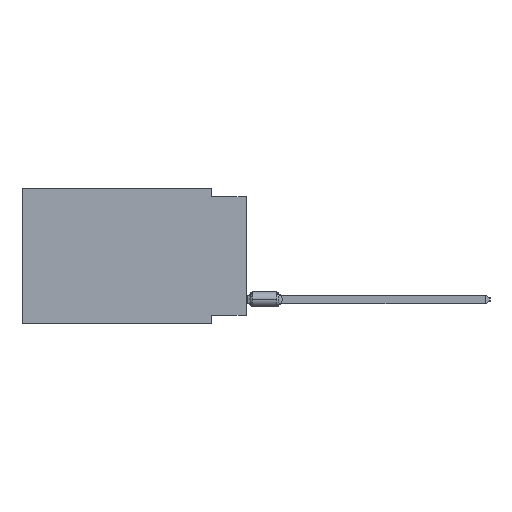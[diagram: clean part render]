
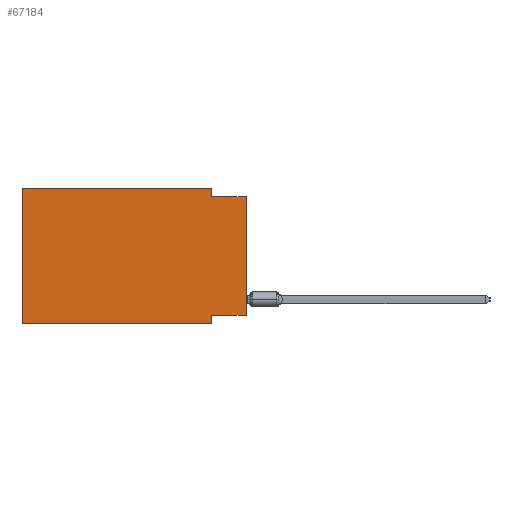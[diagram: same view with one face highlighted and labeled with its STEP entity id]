
A CAD part, left-side view. The second image highlights one B-rep face of the part: STEP entity #67184.
In plain terms, the highlighted planar face has unit normal (-1, 0, 0).
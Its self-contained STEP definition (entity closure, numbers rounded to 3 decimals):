
#1024 = VECTOR ( 'NONE', #66564, 1000. ) ;
#1289 = DIRECTION ( 'NONE',  ( 0., -1., 0. ) ) ;
#3906 = DIRECTION ( 'NONE',  ( 0., 0., -1. ) ) ;
#6473 = DIRECTION ( 'NONE',  ( 0., 0., -1. ) ) ;
#7576 = EDGE_CURVE ( 'NONE', #57149, #52475, #36486, .T. ) ;
#8618 = VECTOR ( 'NONE', #1289, 1000. ) ;
#9998 = CARTESIAN_POINT ( 'NONE',  ( 0., 2.54, -0.635 ) ) ;
#11711 = CARTESIAN_POINT ( 'NONE',  ( 0., 16.383, -9.906 ) ) ;
#12296 = CARTESIAN_POINT ( 'NONE',  ( 0., 16.383, 0. ) ) ;
#13538 = ORIENTED_EDGE ( 'NONE', *, *, #22464, .F. ) ;
#13661 = EDGE_CURVE ( 'NONE', #57149, #59132, #72105, .T. ) ;
#13826 = CARTESIAN_POINT ( 'NONE',  ( 0., 16.383, 0. ) ) ;
#14662 = VERTEX_POINT ( 'NONE', #57443 ) ;
#14938 = VERTEX_POINT ( 'NONE', #66990 ) ;
#15764 = ORIENTED_EDGE ( 'NONE', *, *, #70277, .F. ) ;
#16614 = FACE_OUTER_BOUND ( 'NONE', #52953, .T. ) ;
#16751 = ORIENTED_EDGE ( 'NONE', *, *, #29716, .T. ) ;
#17190 = CARTESIAN_POINT ( 'NONE',  ( 0., 2.54, 0. ) ) ;
#17324 = ORIENTED_EDGE ( 'NONE', *, *, #13661, .T. ) ;
#18807 = PLANE ( 'NONE',  #44376 ) ;
#18891 = EDGE_CURVE ( 'NONE', #14938, #67922, #30468, .T. ) ;
#19079 = ORIENTED_EDGE ( 'NONE', *, *, #30322, .F. ) ;
#22464 = EDGE_CURVE ( 'NONE', #52475, #14662, #55256, .T. ) ;
#22614 = CARTESIAN_POINT ( 'NONE',  ( 0., 2.54, 0. ) ) ;
#24105 = LINE ( 'NONE', #12296, #42124 ) ;
#24469 = DIRECTION ( 'NONE',  ( 0., 0., 1. ) ) ;
#26025 = VERTEX_POINT ( 'NONE', #11711 ) ;
#27175 = CARTESIAN_POINT ( 'NONE',  ( 0., 2.54, -9.906 ) ) ;
#29716 = EDGE_CURVE ( 'NONE', #26025, #14662, #68708, .T. ) ;
#30322 = EDGE_CURVE ( 'NONE', #26025, #14938, #24105, .T. ) ;
#30468 = LINE ( 'NONE', #13826, #8618 ) ;
#33229 = VECTOR ( 'NONE', #58282, 1000. ) ;
#34009 = DIRECTION ( 'NONE',  ( 0., -1., 0. ) ) ;
#34364 = CARTESIAN_POINT ( 'NONE',  ( 0., 16.383, -9.906 ) ) ;
#35000 = VECTOR ( 'NONE', #34009, 1000. ) ;
#35291 = LINE ( 'NONE', #17190, #66000 ) ;
#35441 = CARTESIAN_POINT ( 'NONE',  ( 0., 16.383, 0. ) ) ;
#35893 = VECTOR ( 'NONE', #3906, 1000. ) ;
#36170 = ORIENTED_EDGE ( 'NONE', *, *, #7576, .F. ) ;
#36486 = LINE ( 'NONE', #41662, #33229 ) ;
#37041 = VERTEX_POINT ( 'NONE', #9998 ) ;
#37884 = CARTESIAN_POINT ( 'NONE',  ( 0., 0., -9.271 ) ) ;
#41662 = CARTESIAN_POINT ( 'NONE',  ( 0., 0., -9.271 ) ) ;
#42124 = VECTOR ( 'NONE', #24469, 1000. ) ;
#44376 = AXIS2_PLACEMENT_3D ( 'NONE', #35441, #62791, #57965 ) ;
#49523 = EDGE_CURVE ( 'NONE', #67922, #37041, #35291, .T. ) ;
#52475 = VERTEX_POINT ( 'NONE', #70651 ) ;
#52953 = EDGE_LOOP ( 'NONE', ( #17324, #15764, #55738, #57069, #19079, #16751, #13538, #36170 ) ) ;
#55256 = LINE ( 'NONE', #27175, #35893 ) ;
#55738 = ORIENTED_EDGE ( 'NONE', *, *, #49523, .F. ) ;
#56839 = VECTOR ( 'NONE', #65102, 1000. ) ;
#57069 = ORIENTED_EDGE ( 'NONE', *, *, #18891, .F. ) ;
#57149 = VERTEX_POINT ( 'NONE', #37884 ) ;
#57443 = CARTESIAN_POINT ( 'NONE',  ( 0., 2.54, -9.906 ) ) ;
#57965 = DIRECTION ( 'NONE',  ( 0., 0., -1. ) ) ;
#58282 = DIRECTION ( 'NONE',  ( 0., 1., 0. ) ) ;
#59132 = VERTEX_POINT ( 'NONE', #65795 ) ;
#61022 = LINE ( 'NONE', #66932, #1024 ) ;
#62791 = DIRECTION ( 'NONE',  ( 1., 0., 0. ) ) ;
#65102 = DIRECTION ( 'NONE',  ( 0., 0., 1. ) ) ;
#65795 = CARTESIAN_POINT ( 'NONE',  ( 0., 0., -0.635 ) ) ;
#66000 = VECTOR ( 'NONE', #6473, 1000. ) ;
#66564 = DIRECTION ( 'NONE',  ( 0., -1., 0. ) ) ;
#66932 = CARTESIAN_POINT ( 'NONE',  ( 0., 0., -0.635 ) ) ;
#66990 = CARTESIAN_POINT ( 'NONE',  ( 0., 16.383, 0. ) ) ;
#67184 = ADVANCED_FACE ( 'NONE', ( #16614 ), #18807, .F. ) ;
#67922 = VERTEX_POINT ( 'NONE', #22614 ) ;
#68708 = LINE ( 'NONE', #34364, #35000 ) ;
#70277 = EDGE_CURVE ( 'NONE', #37041, #59132, #61022, .T. ) ;
#70651 = CARTESIAN_POINT ( 'NONE',  ( 0., 2.54, -9.271 ) ) ;
#71376 = CARTESIAN_POINT ( 'NONE',  ( 0., 0., 0. ) ) ;
#72105 = LINE ( 'NONE', #71376, #56839 ) ;
